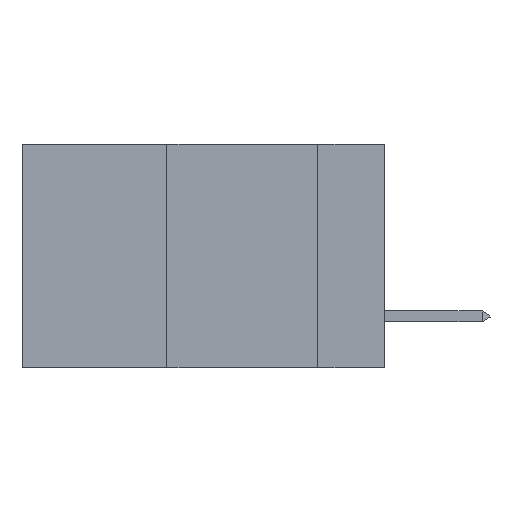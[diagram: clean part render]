
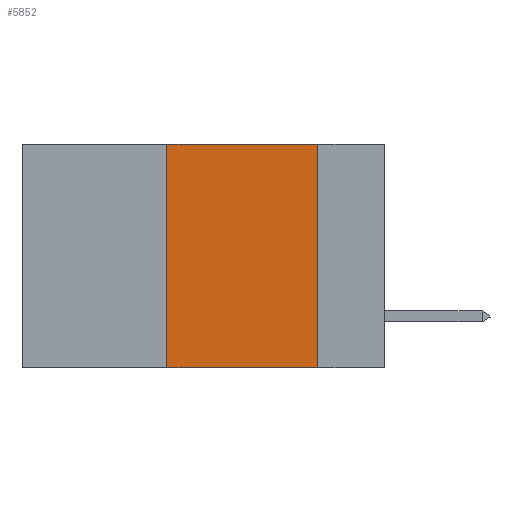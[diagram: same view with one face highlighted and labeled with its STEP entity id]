
A CAD part, left-side view. The second image highlights one B-rep face of the part: STEP entity #5852.
In plain terms, the highlighted planar face has unit normal (-1, 0, 0).
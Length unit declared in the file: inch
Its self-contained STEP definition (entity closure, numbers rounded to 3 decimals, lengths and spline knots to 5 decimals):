
#1108 = LINE ( 'NONE', #15737, #13227 ) ;
#2958 = EDGE_CURVE ( 'NONE', #8654, #7809, #12765, .T. ) ;
#3952 = ORIENTED_EDGE ( 'NONE', *, *, #2958, .F. ) ;
#5127 = VECTOR ( 'NONE', #8885, 39.37008 ) ;
#5341 = ORIENTED_EDGE ( 'NONE', *, *, #9478, .F. ) ;
#5852 = ADVANCED_FACE ( 'NONE', ( #9652 ), #7838, .F. ) ;
#6409 = DIRECTION ( 'NONE',  ( 0., 0., -1. ) ) ;
#6456 = VERTEX_POINT ( 'NONE', #15480 ) ;
#6589 = CARTESIAN_POINT ( 'NONE',  ( 0., 0.36, -0.37 ) ) ;
#6839 = CARTESIAN_POINT ( 'NONE',  ( 0., 0.11, 0. ) ) ;
#7809 = VERTEX_POINT ( 'NONE', #6839 ) ;
#7838 = PLANE ( 'NONE',  #11029 ) ;
#7848 = LINE ( 'NONE', #9040, #5127 ) ;
#8654 = VERTEX_POINT ( 'NONE', #10708 ) ;
#8885 = DIRECTION ( 'NONE',  ( 0., 0., -1. ) ) ;
#9040 = CARTESIAN_POINT ( 'NONE',  ( 0., 0.11, 0. ) ) ;
#9176 = CARTESIAN_POINT ( 'NONE',  ( 0., 0.6, -0.37 ) ) ;
#9478 = EDGE_CURVE ( 'NONE', #10672, #8654, #1108, .T. ) ;
#9652 = FACE_OUTER_BOUND ( 'NONE', #18633, .T. ) ;
#9963 = DIRECTION ( 'NONE',  ( 0., 0., 1. ) ) ;
#10392 = DIRECTION ( 'NONE',  ( 0., -1., 0. ) ) ;
#10513 = LINE ( 'NONE', #9176, #13507 ) ;
#10575 = ORIENTED_EDGE ( 'NONE', *, *, #13670, .T. ) ;
#10672 = VERTEX_POINT ( 'NONE', #6589 ) ;
#10708 = CARTESIAN_POINT ( 'NONE',  ( 0., 0.36, 0. ) ) ;
#10747 = DIRECTION ( 'NONE',  ( 1., 0., 0. ) ) ;
#10791 = DIRECTION ( 'NONE',  ( 0., -1., 0. ) ) ;
#10908 = VECTOR ( 'NONE', #10392, 39.37008 ) ;
#11002 = EDGE_CURVE ( 'NONE', #7809, #6456, #7848, .T. ) ;
#11029 = AXIS2_PLACEMENT_3D ( 'NONE', #13772, #10747, #6409 ) ;
#12765 = LINE ( 'NONE', #18871, #10908 ) ;
#13115 = ORIENTED_EDGE ( 'NONE', *, *, #11002, .F. ) ;
#13227 = VECTOR ( 'NONE', #9963, 39.37008 ) ;
#13507 = VECTOR ( 'NONE', #10791, 39.37008 ) ;
#13670 = EDGE_CURVE ( 'NONE', #10672, #6456, #10513, .T. ) ;
#13772 = CARTESIAN_POINT ( 'NONE',  ( 0., 0.6, 0. ) ) ;
#15480 = CARTESIAN_POINT ( 'NONE',  ( 0., 0.11, -0.37 ) ) ;
#15737 = CARTESIAN_POINT ( 'NONE',  ( 0., 0.36, 0. ) ) ;
#18633 = EDGE_LOOP ( 'NONE', ( #13115, #3952, #5341, #10575 ) ) ;
#18871 = CARTESIAN_POINT ( 'NONE',  ( 0., 0.6, 0. ) ) ;
